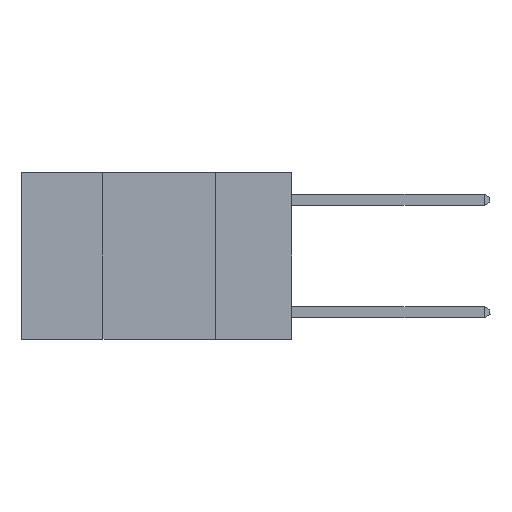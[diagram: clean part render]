
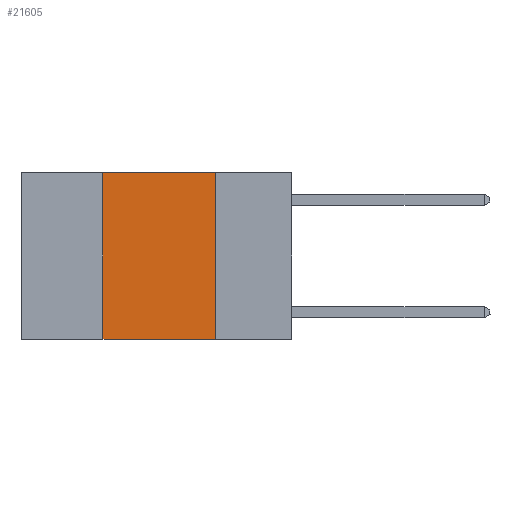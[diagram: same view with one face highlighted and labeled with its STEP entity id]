
A CAD part, left-side view. The second image highlights one B-rep face of the part: STEP entity #21605.
In plain terms, the highlighted planar face has unit normal (-1, 0, 0).
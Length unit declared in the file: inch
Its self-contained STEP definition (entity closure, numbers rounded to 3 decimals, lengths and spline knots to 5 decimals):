
#194 = VECTOR ( 'NONE', #19434, 39.37008 ) ;
#1398 = AXIS2_PLACEMENT_3D ( 'NONE', #16679, #9826, #21653 ) ;
#2083 = VECTOR ( 'NONE', #13795, 39.37008 ) ;
#2649 = VERTEX_POINT ( 'NONE', #19650 ) ;
#2699 = EDGE_LOOP ( 'NONE', ( #8966, #11629, #11675, #12512 ) ) ;
#2842 = VERTEX_POINT ( 'NONE', #18771 ) ;
#4248 = LINE ( 'NONE', #19695, #13780 ) ;
#4785 = EDGE_CURVE ( 'NONE', #2842, #2649, #19891, .T. ) ;
#5760 = EDGE_CURVE ( 'NONE', #2649, #6545, #4248, .T. ) ;
#6185 = VECTOR ( 'NONE', #19314, 39.37008 ) ;
#6545 = VERTEX_POINT ( 'NONE', #6758 ) ;
#6758 = CARTESIAN_POINT ( 'NONE',  ( 0., 0.17, -0.37 ) ) ;
#7809 = DIRECTION ( 'NONE',  ( 0., 0., -1. ) ) ;
#8966 = ORIENTED_EDGE ( 'NONE', *, *, #5760, .F. ) ;
#9826 = DIRECTION ( 'NONE',  ( 1., 0., 0. ) ) ;
#11629 = ORIENTED_EDGE ( 'NONE', *, *, #4785, .F. ) ;
#11675 = ORIENTED_EDGE ( 'NONE', *, *, #13277, .F. ) ;
#11689 = EDGE_CURVE ( 'NONE', #21697, #6545, #18907, .T. ) ;
#12512 = ORIENTED_EDGE ( 'NONE', *, *, #11689, .T. ) ;
#12724 = CARTESIAN_POINT ( 'NONE',  ( 0., 0.6, -0.37 ) ) ;
#13277 = EDGE_CURVE ( 'NONE', #21697, #2842, #17048, .T. ) ;
#13780 = VECTOR ( 'NONE', #7809, 39.37008 ) ;
#13795 = DIRECTION ( 'NONE',  ( 0., 0., 1. ) ) ;
#15177 = CARTESIAN_POINT ( 'NONE',  ( 0., 0.42, -0.37 ) ) ;
#15968 = CARTESIAN_POINT ( 'NONE',  ( 0., 0.6, 0. ) ) ;
#16679 = CARTESIAN_POINT ( 'NONE',  ( 0., 0.6, 0. ) ) ;
#17048 = LINE ( 'NONE', #20462, #2083 ) ;
#18363 = PLANE ( 'NONE',  #1398 ) ;
#18562 = FACE_OUTER_BOUND ( 'NONE', #2699, .T. ) ;
#18771 = CARTESIAN_POINT ( 'NONE',  ( 0., 0.42, 0. ) ) ;
#18907 = LINE ( 'NONE', #12724, #194 ) ;
#19314 = DIRECTION ( 'NONE',  ( 0., -1., 0. ) ) ;
#19434 = DIRECTION ( 'NONE',  ( 0., -1., 0. ) ) ;
#19650 = CARTESIAN_POINT ( 'NONE',  ( 0., 0.17, 0. ) ) ;
#19695 = CARTESIAN_POINT ( 'NONE',  ( 0., 0.17, 0. ) ) ;
#19891 = LINE ( 'NONE', #15968, #6185 ) ;
#20462 = CARTESIAN_POINT ( 'NONE',  ( 0., 0.42, 0. ) ) ;
#21605 = ADVANCED_FACE ( 'NONE', ( #18562 ), #18363, .F. ) ;
#21653 = DIRECTION ( 'NONE',  ( 0., 0., -1. ) ) ;
#21697 = VERTEX_POINT ( 'NONE', #15177 ) ;
